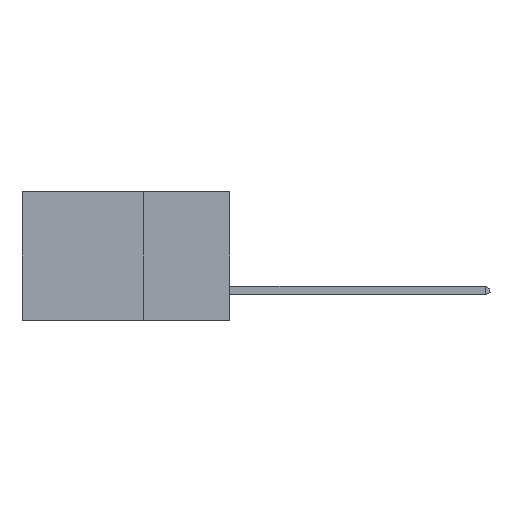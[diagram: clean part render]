
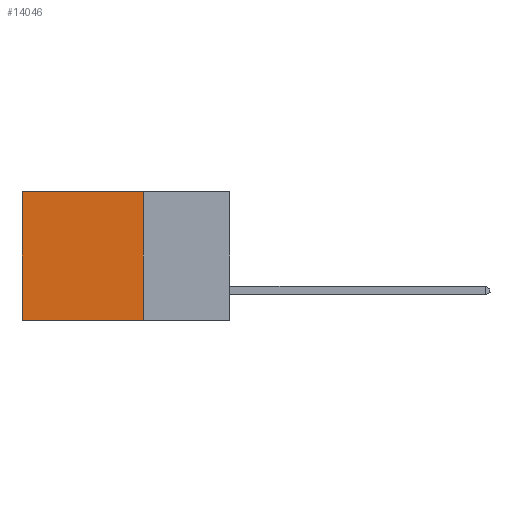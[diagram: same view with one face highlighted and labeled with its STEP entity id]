
A CAD part, left-side view. The second image highlights one B-rep face of the part: STEP entity #14046.
In plain terms, the highlighted planar face has unit normal (-1, 0, 0).
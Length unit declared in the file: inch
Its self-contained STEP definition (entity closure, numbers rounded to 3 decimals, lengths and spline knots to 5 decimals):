
#90 = VERTEX_POINT ( 'NONE', #18812 ) ;
#284 = CARTESIAN_POINT ( 'NONE',  ( 0.298, 0.6, 0. ) ) ;
#665 = EDGE_CURVE ( 'NONE', #90, #7408, #19324, .T. ) ;
#1372 = CARTESIAN_POINT ( 'NONE',  ( 0.298, 0.6, -0.37 ) ) ;
#1662 = CARTESIAN_POINT ( 'NONE',  ( 0.298, 0.25, -0.37 ) ) ;
#2835 = VECTOR ( 'NONE', #10009, 39.37008 ) ;
#3247 = CARTESIAN_POINT ( 'NONE',  ( 0.298, 0.25, 0. ) ) ;
#3817 = CARTESIAN_POINT ( 'NONE',  ( 0.298, 0.25, 0. ) ) ;
#3893 = PLANE ( 'NONE',  #14763 ) ;
#4114 = DIRECTION ( 'NONE',  ( 0., 0., -1. ) ) ;
#5602 = EDGE_LOOP ( 'NONE', ( #7382, #7257, #7570, #19571 ) ) ;
#7257 = ORIENTED_EDGE ( 'NONE', *, *, #665, .F. ) ;
#7382 = ORIENTED_EDGE ( 'NONE', *, *, #14417, .T. ) ;
#7408 = VERTEX_POINT ( 'NONE', #1372 ) ;
#7570 = ORIENTED_EDGE ( 'NONE', *, *, #19570, .F. ) ;
#10009 = DIRECTION ( 'NONE',  ( 0., 0., -1. ) ) ;
#10106 = FACE_OUTER_BOUND ( 'NONE', #5602, .T. ) ;
#10481 = LINE ( 'NONE', #22107, #18261 ) ;
#11483 = LINE ( 'NONE', #20682, #2835 ) ;
#11777 = DIRECTION ( 'NONE',  ( 0., 1., 0. ) ) ;
#11790 = VECTOR ( 'NONE', #19445, 39.37008 ) ;
#13034 = EDGE_CURVE ( 'NONE', #16475, #20791, #10481, .T. ) ;
#14046 = ADVANCED_FACE ( 'NONE', ( #10106 ), #3893, .F. ) ;
#14417 = EDGE_CURVE ( 'NONE', #20791, #7408, #11483, .T. ) ;
#14763 = AXIS2_PLACEMENT_3D ( 'NONE', #3817, #14784, #4114 ) ;
#14784 = DIRECTION ( 'NONE',  ( 1., 0., 0. ) ) ;
#15154 = VECTOR ( 'NONE', #19073, 39.37008 ) ;
#15364 = CARTESIAN_POINT ( 'NONE',  ( 0.298, 0.25, 0. ) ) ;
#16475 = VERTEX_POINT ( 'NONE', #3247 ) ;
#18261 = VECTOR ( 'NONE', #11777, 39.37008 ) ;
#18812 = CARTESIAN_POINT ( 'NONE',  ( 0.298, 0.25, -0.37 ) ) ;
#19073 = DIRECTION ( 'NONE',  ( 0., 0., -1. ) ) ;
#19324 = LINE ( 'NONE', #1662, #11790 ) ;
#19336 = LINE ( 'NONE', #15364, #15154 ) ;
#19445 = DIRECTION ( 'NONE',  ( 0., 1., 0. ) ) ;
#19570 = EDGE_CURVE ( 'NONE', #16475, #90, #19336, .T. ) ;
#19571 = ORIENTED_EDGE ( 'NONE', *, *, #13034, .T. ) ;
#20682 = CARTESIAN_POINT ( 'NONE',  ( 0.298, 0.6, 0. ) ) ;
#20791 = VERTEX_POINT ( 'NONE', #284 ) ;
#22107 = CARTESIAN_POINT ( 'NONE',  ( 0.298, 0.25, 0. ) ) ;
